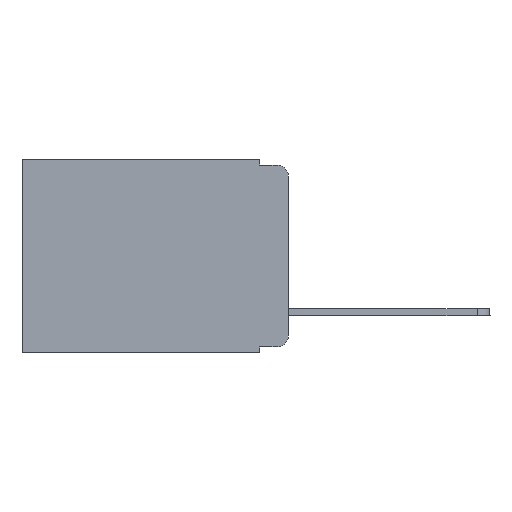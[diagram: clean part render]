
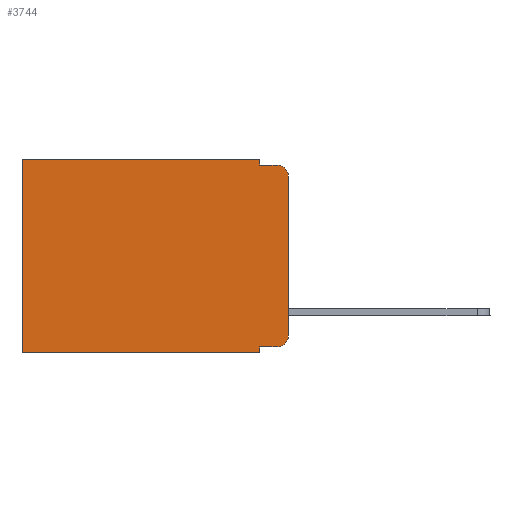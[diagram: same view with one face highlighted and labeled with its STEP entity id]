
A CAD part, left-side view. The second image highlights one B-rep face of the part: STEP entity #3744.
In plain terms, the highlighted planar face has unit normal (-1, 0, 0).
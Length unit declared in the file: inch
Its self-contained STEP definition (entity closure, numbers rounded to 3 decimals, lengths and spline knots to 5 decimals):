
#4 = ORIENTED_EDGE ( 'NONE', *, *, #6370, .T. ) ;
#81 = VERTEX_POINT ( 'NONE', #6317 ) ;
#94 = ORIENTED_EDGE ( 'NONE', *, *, #1177, .T. ) ;
#216 = CARTESIAN_POINT ( 'NONE',  ( 0.298, 0.473, 0. ) ) ;
#362 = ORIENTED_EDGE ( 'NONE', *, *, #5846, .F. ) ;
#595 = CARTESIAN_POINT ( 'NONE',  ( 0.298, 0.051, -0.333 ) ) ;
#1177 = EDGE_CURVE ( 'NONE', #8651, #10725, #4384, .T. ) ;
#1404 = LINE ( 'NONE', #3751, #7504 ) ;
#2191 = DIRECTION ( 'NONE',  ( 1., 0., 0. ) ) ;
#2325 = CARTESIAN_POINT ( 'NONE',  ( 0.298, 0.02, -0.03 ) ) ;
#2834 = VECTOR ( 'NONE', #7361, 39.37008 ) ;
#2939 = CARTESIAN_POINT ( 'NONE',  ( 0.298, 0.051, 0. ) ) ;
#3261 = CARTESIAN_POINT ( 'NONE',  ( 0.298, 0.02, -0.313 ) ) ;
#3744 = ADVANCED_FACE ( 'NONE', ( #7157 ), #12111, .F. ) ;
#3751 = CARTESIAN_POINT ( 'NONE',  ( 0.298, 0.051, -0.01 ) ) ;
#3882 = EDGE_CURVE ( 'NONE', #4638, #9353, #1404, .T. ) ;
#4384 = LINE ( 'NONE', #216, #2834 ) ;
#4548 = VECTOR ( 'NONE', #11309, 39.37008 ) ;
#4638 = VERTEX_POINT ( 'NONE', #15220 ) ;
#5075 = VECTOR ( 'NONE', #6679, 39.37008 ) ;
#5135 = CARTESIAN_POINT ( 'NONE',  ( 0.298, 0.051, -0.343 ) ) ;
#5238 = EDGE_CURVE ( 'NONE', #7323, #9353, #7350, .T. ) ;
#5284 = CARTESIAN_POINT ( 'NONE',  ( 0.298, 0.473, 0. ) ) ;
#5302 = EDGE_CURVE ( 'NONE', #14597, #81, #14475, .T. ) ;
#5493 = LINE ( 'NONE', #2939, #4548 ) ;
#5728 = CARTESIAN_POINT ( 'NONE',  ( 0.298, 0., 0. ) ) ;
#5794 = ORIENTED_EDGE ( 'NONE', *, *, #7661, .F. ) ;
#5802 = CARTESIAN_POINT ( 'NONE',  ( 0.298, 0., -0.343 ) ) ;
#5846 = EDGE_CURVE ( 'NONE', #7749, #10725, #12132, .T. ) ;
#6191 = AXIS2_PLACEMENT_3D ( 'NONE', #14384, #2191, #13355 ) ;
#6317 = CARTESIAN_POINT ( 'NONE',  ( 0.298, 0.02, -0.333 ) ) ;
#6370 = EDGE_CURVE ( 'NONE', #11875, #8651, #12901, .T. ) ;
#6623 = AXIS2_PLACEMENT_3D ( 'NONE', #3261, #7979, #13015 ) ;
#6629 = EDGE_LOOP ( 'NONE', ( #5794, #8028, #12683, #11172, #4, #94, #362, #14057, #9930, #12624 ) ) ;
#6679 = DIRECTION ( 'NONE',  ( 0., -1., 0. ) ) ;
#7121 = CARTESIAN_POINT ( 'NONE',  ( 0.298, 0.051, -0.333 ) ) ;
#7157 = FACE_OUTER_BOUND ( 'NONE', #6629, .T. ) ;
#7323 = VERTEX_POINT ( 'NONE', #8317 ) ;
#7350 = CIRCLE ( 'NONE', #10334, 0.02 ) ;
#7361 = DIRECTION ( 'NONE',  ( 0., 0., -1. ) ) ;
#7390 = CARTESIAN_POINT ( 'NONE',  ( 0.298, 0., -0.313 ) ) ;
#7504 = VECTOR ( 'NONE', #8569, 39.37008 ) ;
#7661 = EDGE_CURVE ( 'NONE', #7323, #10043, #15752, .T. ) ;
#7749 = VERTEX_POINT ( 'NONE', #5135 ) ;
#7979 = DIRECTION ( 'NONE',  ( -1., 0., 0. ) ) ;
#8028 = ORIENTED_EDGE ( 'NONE', *, *, #5238, .T. ) ;
#8107 = VECTOR ( 'NONE', #10645, 39.37008 ) ;
#8317 = CARTESIAN_POINT ( 'NONE',  ( 0.298, 0., -0.03 ) ) ;
#8553 = DIRECTION ( 'NONE',  ( 0., 0., -1. ) ) ;
#8569 = DIRECTION ( 'NONE',  ( 0., -1., 0. ) ) ;
#8651 = VERTEX_POINT ( 'NONE', #5284 ) ;
#9237 = VECTOR ( 'NONE', #15882, 39.37008 ) ;
#9248 = CIRCLE ( 'NONE', #6623, 0.02 ) ;
#9353 = VERTEX_POINT ( 'NONE', #12152 ) ;
#9930 = ORIENTED_EDGE ( 'NONE', *, *, #5302, .T. ) ;
#10043 = VERTEX_POINT ( 'NONE', #7390 ) ;
#10334 = AXIS2_PLACEMENT_3D ( 'NONE', #2325, #12094, #8553 ) ;
#10379 = CARTESIAN_POINT ( 'NONE',  ( 0.298, 0.051, 0. ) ) ;
#10387 = CARTESIAN_POINT ( 'NONE',  ( 0.298, 0.051, 0. ) ) ;
#10645 = DIRECTION ( 'NONE',  ( 0., 1., 0. ) ) ;
#10725 = VERTEX_POINT ( 'NONE', #12802 ) ;
#11103 = EDGE_CURVE ( 'NONE', #11875, #4638, #5493, .T. ) ;
#11148 = VECTOR ( 'NONE', #14486, 39.37008 ) ;
#11172 = ORIENTED_EDGE ( 'NONE', *, *, #11103, .F. ) ;
#11309 = DIRECTION ( 'NONE',  ( 0., 0., -1. ) ) ;
#11780 = DIRECTION ( 'NONE',  ( 0., 0., -1. ) ) ;
#11875 = VERTEX_POINT ( 'NONE', #10379 ) ;
#12094 = DIRECTION ( 'NONE',  ( -1., 0., 0. ) ) ;
#12111 = PLANE ( 'NONE',  #6191 ) ;
#12132 = LINE ( 'NONE', #5802, #11148 ) ;
#12152 = CARTESIAN_POINT ( 'NONE',  ( 0.298, 0.02, -0.01 ) ) ;
#12624 = ORIENTED_EDGE ( 'NONE', *, *, #13728, .T. ) ;
#12683 = ORIENTED_EDGE ( 'NONE', *, *, #3882, .F. ) ;
#12802 = CARTESIAN_POINT ( 'NONE',  ( 0.298, 0.473, -0.343 ) ) ;
#12901 = LINE ( 'NONE', #5728, #8107 ) ;
#13015 = DIRECTION ( 'NONE',  ( 0., 0., -1. ) ) ;
#13227 = VECTOR ( 'NONE', #11780, 39.37008 ) ;
#13355 = DIRECTION ( 'NONE',  ( 0., 0., -1. ) ) ;
#13391 = CARTESIAN_POINT ( 'NONE',  ( 0.298, 0., 0. ) ) ;
#13728 = EDGE_CURVE ( 'NONE', #81, #10043, #9248, .T. ) ;
#14057 = ORIENTED_EDGE ( 'NONE', *, *, #14444, .F. ) ;
#14384 = CARTESIAN_POINT ( 'NONE',  ( 0.298, 0., 0. ) ) ;
#14444 = EDGE_CURVE ( 'NONE', #14597, #7749, #14751, .T. ) ;
#14475 = LINE ( 'NONE', #595, #5075 ) ;
#14486 = DIRECTION ( 'NONE',  ( 0., 1., 0. ) ) ;
#14597 = VERTEX_POINT ( 'NONE', #7121 ) ;
#14751 = LINE ( 'NONE', #10387, #13227 ) ;
#15220 = CARTESIAN_POINT ( 'NONE',  ( 0.298, 0.051, -0.01 ) ) ;
#15752 = LINE ( 'NONE', #13391, #9237 ) ;
#15882 = DIRECTION ( 'NONE',  ( 0., 0., -1. ) ) ;
